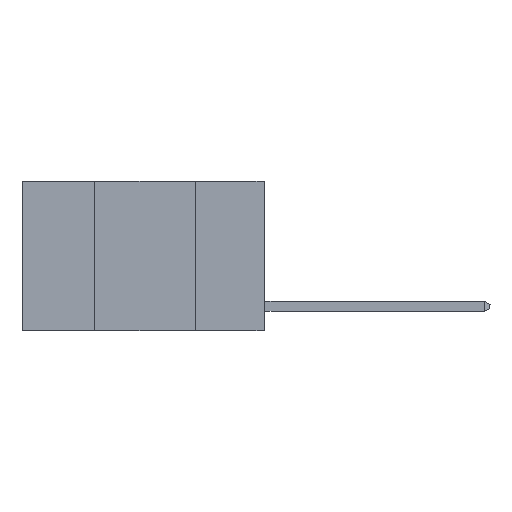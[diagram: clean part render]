
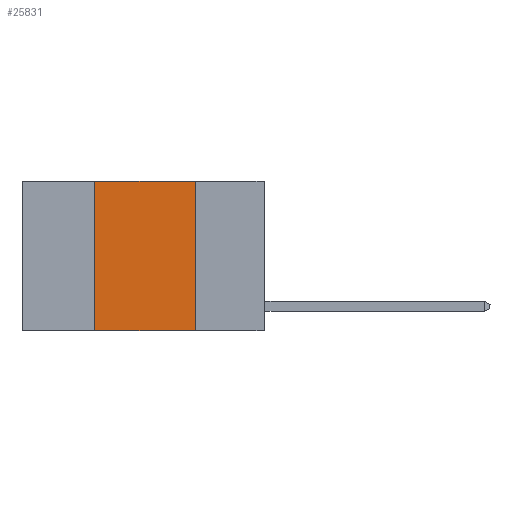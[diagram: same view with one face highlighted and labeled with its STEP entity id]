
A CAD part, left-side view. The second image highlights one B-rep face of the part: STEP entity #25831.
In plain terms, the highlighted planar face has unit normal (-1, 0, 0).
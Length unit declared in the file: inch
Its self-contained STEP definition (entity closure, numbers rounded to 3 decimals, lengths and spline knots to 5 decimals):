
#104 = ORIENTED_EDGE ( 'NONE', *, *, #18957, .T. ) ;
#1018 = VERTEX_POINT ( 'NONE', #16238 ) ;
#1932 = CARTESIAN_POINT ( 'NONE',  ( 0., 0.6, -0.37 ) ) ;
#2278 = VECTOR ( 'NONE', #10017, 39.37008 ) ;
#2388 = CARTESIAN_POINT ( 'NONE',  ( 0., 0.42, 0. ) ) ;
#3393 = CARTESIAN_POINT ( 'NONE',  ( 0., 0.17, 0. ) ) ;
#3653 = LINE ( 'NONE', #3393, #5547 ) ;
#4495 = ORIENTED_EDGE ( 'NONE', *, *, #12722, .F. ) ;
#5328 = CARTESIAN_POINT ( 'NONE',  ( 0., 0.17, -0.37 ) ) ;
#5547 = VECTOR ( 'NONE', #17789, 39.37008 ) ;
#7019 = VECTOR ( 'NONE', #20083, 39.37008 ) ;
#8177 = VERTEX_POINT ( 'NONE', #16904 ) ;
#10017 = DIRECTION ( 'NONE',  ( 0., -1., 0. ) ) ;
#10036 = CARTESIAN_POINT ( 'NONE',  ( 0., 0.42, 0. ) ) ;
#12017 = LINE ( 'NONE', #10036, #7019 ) ;
#12653 = LINE ( 'NONE', #1932, #2278 ) ;
#12722 = EDGE_CURVE ( 'NONE', #14753, #1018, #15375, .T. ) ;
#14753 = VERTEX_POINT ( 'NONE', #2388 ) ;
#15375 = LINE ( 'NONE', #25312, #22695 ) ;
#16000 = CARTESIAN_POINT ( 'NONE',  ( 0., 0.6, 0. ) ) ;
#16143 = EDGE_CURVE ( 'NONE', #1018, #20493, #3653, .T. ) ;
#16238 = CARTESIAN_POINT ( 'NONE',  ( 0., 0.17, 0. ) ) ;
#16904 = CARTESIAN_POINT ( 'NONE',  ( 0., 0.42, -0.37 ) ) ;
#17789 = DIRECTION ( 'NONE',  ( 0., 0., -1. ) ) ;
#18554 = ORIENTED_EDGE ( 'NONE', *, *, #16143, .F. ) ;
#18702 = EDGE_LOOP ( 'NONE', ( #18554, #4495, #21428, #104 ) ) ;
#18957 = EDGE_CURVE ( 'NONE', #8177, #20493, #12653, .T. ) ;
#19971 = FACE_OUTER_BOUND ( 'NONE', #18702, .T. ) ;
#20083 = DIRECTION ( 'NONE',  ( 0., 0., 1. ) ) ;
#20493 = VERTEX_POINT ( 'NONE', #5328 ) ;
#21428 = ORIENTED_EDGE ( 'NONE', *, *, #22915, .F. ) ;
#21954 = PLANE ( 'NONE',  #23970 ) ;
#22082 = DIRECTION ( 'NONE',  ( 0., 0., -1. ) ) ;
#22695 = VECTOR ( 'NONE', #25571, 39.37008 ) ;
#22915 = EDGE_CURVE ( 'NONE', #8177, #14753, #12017, .T. ) ;
#23970 = AXIS2_PLACEMENT_3D ( 'NONE', #16000, #24341, #22082 ) ;
#24341 = DIRECTION ( 'NONE',  ( 1., 0., 0. ) ) ;
#25312 = CARTESIAN_POINT ( 'NONE',  ( 0., 0.6, 0. ) ) ;
#25571 = DIRECTION ( 'NONE',  ( 0., -1., 0. ) ) ;
#25831 = ADVANCED_FACE ( 'NONE', ( #19971 ), #21954, .F. ) ;
